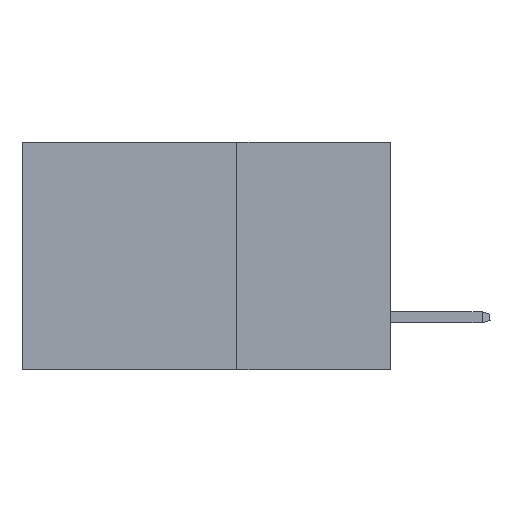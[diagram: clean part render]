
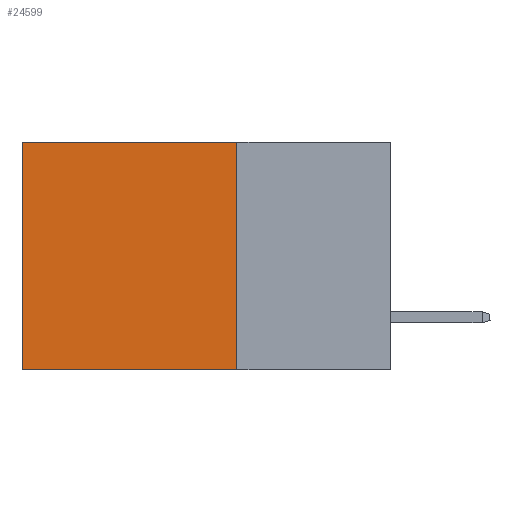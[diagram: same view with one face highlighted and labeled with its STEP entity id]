
A CAD part, left-side view. The second image highlights one B-rep face of the part: STEP entity #24599.
In plain terms, the highlighted planar face has unit normal (-1, 0, 0).
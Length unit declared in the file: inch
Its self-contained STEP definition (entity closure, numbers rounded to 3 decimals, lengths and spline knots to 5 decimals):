
#1517 = VECTOR ( 'NONE', #30898, 39.37008 ) ;
#2901 = EDGE_CURVE ( 'NONE', #5953, #13419, #31003, .T. ) ;
#5572 = DIRECTION ( 'NONE',  ( 0., 0., -1. ) ) ;
#5719 = LINE ( 'NONE', #21184, #23094 ) ;
#5741 = VERTEX_POINT ( 'NONE', #25518 ) ;
#5791 = DIRECTION ( 'NONE',  ( 1., 0., 0. ) ) ;
#5953 = VERTEX_POINT ( 'NONE', #29620 ) ;
#6327 = EDGE_CURVE ( 'NONE', #23326, #5741, #29648, .T. ) ;
#7526 = FACE_OUTER_BOUND ( 'NONE', #21788, .T. ) ;
#7843 = ORIENTED_EDGE ( 'NONE', *, *, #20917, .T. ) ;
#10322 = ORIENTED_EDGE ( 'NONE', *, *, #6327, .F. ) ;
#10700 = DIRECTION ( 'NONE',  ( 0., 1., 0. ) ) ;
#11495 = CARTESIAN_POINT ( 'NONE',  ( 0.2875, 0.6, -0.37 ) ) ;
#12559 = VECTOR ( 'NONE', #5572, 39.37008 ) ;
#13419 = VERTEX_POINT ( 'NONE', #11495 ) ;
#15087 = EDGE_CURVE ( 'NONE', #5741, #13419, #17816, .T. ) ;
#17330 = ORIENTED_EDGE ( 'NONE', *, *, #15087, .F. ) ;
#17816 = LINE ( 'NONE', #30737, #1517 ) ;
#18018 = PLANE ( 'NONE',  #23344 ) ;
#20169 = CARTESIAN_POINT ( 'NONE',  ( 0.2875, 0.6, 0. ) ) ;
#20758 = DIRECTION ( 'NONE',  ( 0., 0., -1. ) ) ;
#20917 = EDGE_CURVE ( 'NONE', #23326, #5953, #5719, .T. ) ;
#21184 = CARTESIAN_POINT ( 'NONE',  ( 0.2875, 0.25, 0. ) ) ;
#21788 = EDGE_LOOP ( 'NONE', ( #28832, #17330, #10322, #7843 ) ) ;
#22854 = VECTOR ( 'NONE', #33420, 39.37008 ) ;
#23094 = VECTOR ( 'NONE', #10700, 39.37008 ) ;
#23326 = VERTEX_POINT ( 'NONE', #25765 ) ;
#23344 = AXIS2_PLACEMENT_3D ( 'NONE', #29351, #5791, #20758 ) ;
#24599 = ADVANCED_FACE ( 'NONE', ( #7526 ), #18018, .F. ) ;
#24658 = CARTESIAN_POINT ( 'NONE',  ( 0.2875, 0.25, 0. ) ) ;
#25518 = CARTESIAN_POINT ( 'NONE',  ( 0.2875, 0.25, -0.37 ) ) ;
#25765 = CARTESIAN_POINT ( 'NONE',  ( 0.2875, 0.25, 0. ) ) ;
#28832 = ORIENTED_EDGE ( 'NONE', *, *, #2901, .T. ) ;
#29351 = CARTESIAN_POINT ( 'NONE',  ( 0.2875, 0.25, 0. ) ) ;
#29620 = CARTESIAN_POINT ( 'NONE',  ( 0.2875, 0.6, 0. ) ) ;
#29648 = LINE ( 'NONE', #24658, #12559 ) ;
#30737 = CARTESIAN_POINT ( 'NONE',  ( 0.2875, 0.25, -0.37 ) ) ;
#30898 = DIRECTION ( 'NONE',  ( 0., 1., 0. ) ) ;
#31003 = LINE ( 'NONE', #20169, #22854 ) ;
#33420 = DIRECTION ( 'NONE',  ( 0., 0., -1. ) ) ;
